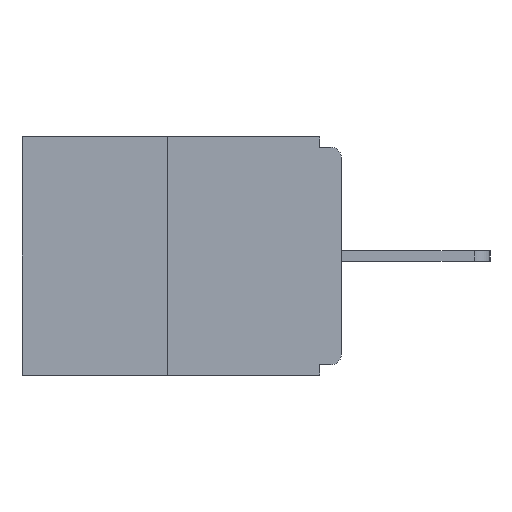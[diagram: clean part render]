
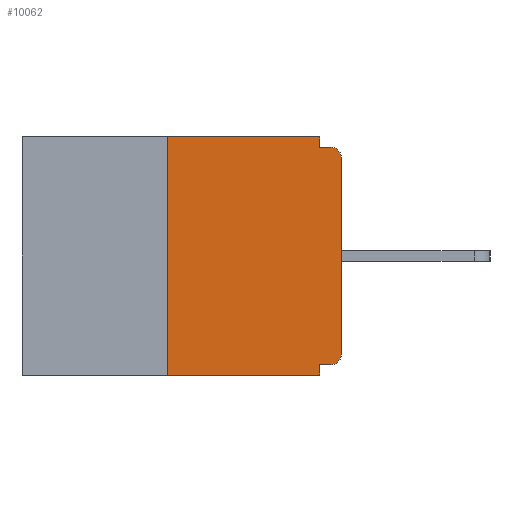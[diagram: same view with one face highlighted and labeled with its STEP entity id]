
A CAD part, left-side view. The second image highlights one B-rep face of the part: STEP entity #10062.
In plain terms, the highlighted planar face has unit normal (-1, 0, 0).
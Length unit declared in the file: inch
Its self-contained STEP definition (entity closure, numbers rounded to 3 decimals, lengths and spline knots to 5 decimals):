
#201 = CARTESIAN_POINT ( 'NONE',  ( 0., 0.031, -0.343 ) ) ;
#375 = CARTESIAN_POINT ( 'NONE',  ( 0., 0.031, -0.015 ) ) ;
#443 = EDGE_CURVE ( 'NONE', #3547, #2870, #3043, .T. ) ;
#602 = LINE ( 'NONE', #12967, #11876 ) ;
#992 = DIRECTION ( 'NONE',  ( 0., -1., 0. ) ) ;
#1238 = EDGE_CURVE ( 'NONE', #1356, #1842, #5562, .T. ) ;
#1356 = VERTEX_POINT ( 'NONE', #2101 ) ;
#1842 = VERTEX_POINT ( 'NONE', #6637 ) ;
#1990 = DIRECTION ( 'NONE',  ( 0., 0., -1. ) ) ;
#2101 = CARTESIAN_POINT ( 'NONE',  ( 0., 0., -0.03 ) ) ;
#2738 = EDGE_CURVE ( 'NONE', #2870, #12223, #3948, .T. ) ;
#2828 = DIRECTION ( 'NONE',  ( 0., 1., 0. ) ) ;
#2870 = VERTEX_POINT ( 'NONE', #4932 ) ;
#2930 = CARTESIAN_POINT ( 'NONE',  ( 0., 0.25, -0.343 ) ) ;
#3043 = LINE ( 'NONE', #7201, #10875 ) ;
#3149 = CARTESIAN_POINT ( 'NONE',  ( 0., 0.46, 0. ) ) ;
#3501 = EDGE_CURVE ( 'NONE', #9450, #4284, #8424, .T. ) ;
#3529 = ORIENTED_EDGE ( 'NONE', *, *, #443, .F. ) ;
#3547 = VERTEX_POINT ( 'NONE', #6855 ) ;
#3570 = ORIENTED_EDGE ( 'NONE', *, *, #7178, .F. ) ;
#3575 = ORIENTED_EDGE ( 'NONE', *, *, #5671, .T. ) ;
#3601 = ORIENTED_EDGE ( 'NONE', *, *, #3501, .F. ) ;
#3637 = ORIENTED_EDGE ( 'NONE', *, *, #9494, .F. ) ;
#3732 = CARTESIAN_POINT ( 'NONE',  ( 0., 0.25, 0. ) ) ;
#3782 = ORIENTED_EDGE ( 'NONE', *, *, #4383, .T. ) ;
#3796 = ORIENTED_EDGE ( 'NONE', *, *, #13240, .T. ) ;
#3864 = ORIENTED_EDGE ( 'NONE', *, *, #1238, .T. ) ;
#3918 = ORIENTED_EDGE ( 'NONE', *, *, #5856, .F. ) ;
#3948 = LINE ( 'NONE', #8896, #6514 ) ;
#3964 = ORIENTED_EDGE ( 'NONE', *, *, #2738, .F. ) ;
#4284 = VERTEX_POINT ( 'NONE', #201 ) ;
#4383 = EDGE_CURVE ( 'NONE', #12102, #10609, #10781, .T. ) ;
#4397 = VECTOR ( 'NONE', #4965, 39.37008 ) ;
#4543 = EDGE_LOOP ( 'NONE', ( #3529, #3570, #3575, #3601, #3637, #3782, #3796, #3864, #3918, #3964 ) ) ;
#4932 = CARTESIAN_POINT ( 'NONE',  ( 0., 0.031, 0. ) ) ;
#4965 = DIRECTION ( 'NONE',  ( 0., -1., 0. ) ) ;
#5232 = VECTOR ( 'NONE', #992, 39.37008 ) ;
#5443 = DIRECTION ( 'NONE',  ( 0., 0., -1. ) ) ;
#5478 = DIRECTION ( 'NONE',  ( -1., 0., 0. ) ) ;
#5562 = CIRCLE ( 'NONE', #6087, 0.015 ) ;
#5671 = EDGE_CURVE ( 'NONE', #11813, #4284, #10148, .T. ) ;
#5733 = AXIS2_PLACEMENT_3D ( 'NONE', #13772, #5478, #5443 ) ;
#5856 = EDGE_CURVE ( 'NONE', #12223, #1842, #8550, .T. ) ;
#5908 = DIRECTION ( 'NONE',  ( 0., 0., 1. ) ) ;
#6087 = AXIS2_PLACEMENT_3D ( 'NONE', #9362, #13304, #8330 ) ;
#6514 = VECTOR ( 'NONE', #12080, 39.37008 ) ;
#6575 = AXIS2_PLACEMENT_3D ( 'NONE', #3149, #8664, #1990 ) ;
#6637 = CARTESIAN_POINT ( 'NONE',  ( 0., 0.015, -0.015 ) ) ;
#6651 = DIRECTION ( 'NONE',  ( 0., 0., -1. ) ) ;
#6855 = CARTESIAN_POINT ( 'NONE',  ( 0., 0.25, 0. ) ) ;
#7126 = CARTESIAN_POINT ( 'NONE',  ( 0., 0.031, -0.343 ) ) ;
#7178 = EDGE_CURVE ( 'NONE', #11813, #3547, #8342, .T. ) ;
#7179 = DIRECTION ( 'NONE',  ( 0., -1., 0. ) ) ;
#7201 = CARTESIAN_POINT ( 'NONE',  ( 0., 0.46, 0. ) ) ;
#7581 = PLANE ( 'NONE',  #6575 ) ;
#8193 = DIRECTION ( 'NONE',  ( 0., 0., 1. ) ) ;
#8330 = DIRECTION ( 'NONE',  ( 0., 0., -1. ) ) ;
#8342 = LINE ( 'NONE', #3732, #10981 ) ;
#8424 = LINE ( 'NONE', #7126, #13188 ) ;
#8550 = LINE ( 'NONE', #10963, #5232 ) ;
#8664 = DIRECTION ( 'NONE',  ( 1., 0., 0. ) ) ;
#8896 = CARTESIAN_POINT ( 'NONE',  ( 0., 0.031, 0. ) ) ;
#9342 = CARTESIAN_POINT ( 'NONE',  ( 0., 0., -0.328 ) ) ;
#9362 = CARTESIAN_POINT ( 'NONE',  ( 0., 0.015, -0.03 ) ) ;
#9445 = CARTESIAN_POINT ( 'NONE',  ( 0., 0., -0.313 ) ) ;
#9450 = VERTEX_POINT ( 'NONE', #12996 ) ;
#9494 = EDGE_CURVE ( 'NONE', #12102, #9450, #12937, .T. ) ;
#10062 = ADVANCED_FACE ( 'NONE', ( #12899 ), #7581, .F. ) ;
#10148 = LINE ( 'NONE', #10991, #4397 ) ;
#10609 = VERTEX_POINT ( 'NONE', #9445 ) ;
#10781 = CIRCLE ( 'NONE', #5733, 0.015 ) ;
#10875 = VECTOR ( 'NONE', #7179, 39.37008 ) ;
#10963 = CARTESIAN_POINT ( 'NONE',  ( 0., 0., -0.015 ) ) ;
#10981 = VECTOR ( 'NONE', #5908, 39.37008 ) ;
#10991 = CARTESIAN_POINT ( 'NONE',  ( 0., 0.46, -0.343 ) ) ;
#11275 = CARTESIAN_POINT ( 'NONE',  ( 0., 0.015, -0.328 ) ) ;
#11813 = VERTEX_POINT ( 'NONE', #2930 ) ;
#11876 = VECTOR ( 'NONE', #8193, 39.37008 ) ;
#12080 = DIRECTION ( 'NONE',  ( 0., 0., -1. ) ) ;
#12102 = VERTEX_POINT ( 'NONE', #11275 ) ;
#12223 = VERTEX_POINT ( 'NONE', #375 ) ;
#12899 = FACE_OUTER_BOUND ( 'NONE', #4543, .T. ) ;
#12937 = LINE ( 'NONE', #9342, #13215 ) ;
#12967 = CARTESIAN_POINT ( 'NONE',  ( 0., 0., 0. ) ) ;
#12996 = CARTESIAN_POINT ( 'NONE',  ( 0., 0.031, -0.328 ) ) ;
#13188 = VECTOR ( 'NONE', #6651, 39.37008 ) ;
#13215 = VECTOR ( 'NONE', #2828, 39.37008 ) ;
#13240 = EDGE_CURVE ( 'NONE', #10609, #1356, #602, .T. ) ;
#13304 = DIRECTION ( 'NONE',  ( -1., 0., 0. ) ) ;
#13772 = CARTESIAN_POINT ( 'NONE',  ( 0., 0.015, -0.313 ) ) ;
